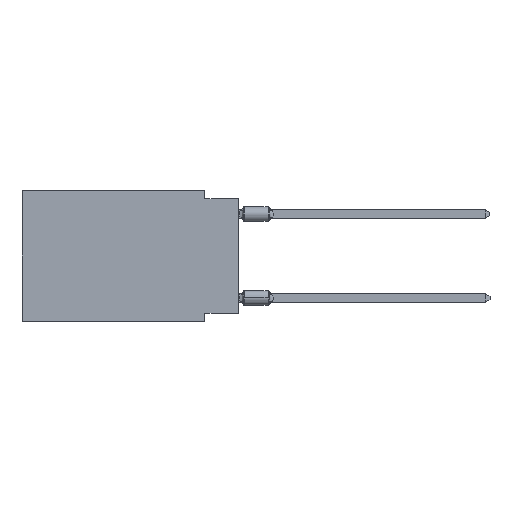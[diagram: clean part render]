
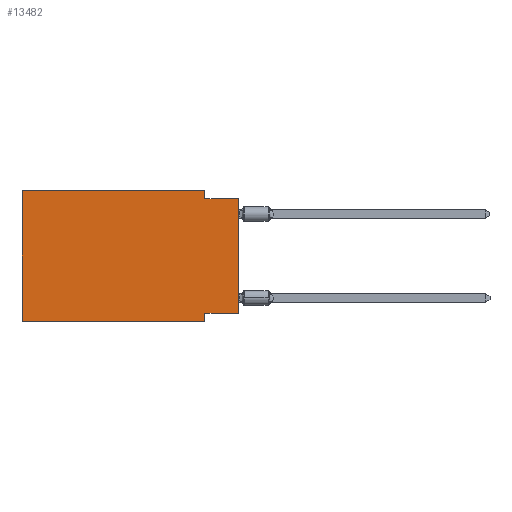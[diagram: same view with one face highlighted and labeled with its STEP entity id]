
A CAD part, left-side view. The second image highlights one B-rep face of the part: STEP entity #13482.
In plain terms, the highlighted planar face has unit normal (-1, 0, 0).
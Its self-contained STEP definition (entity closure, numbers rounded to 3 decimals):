
#192 = VECTOR ( 'NONE', #12420, 1000. ) ;
#428 = FACE_OUTER_BOUND ( 'NONE', #1372, .T. ) ;
#1372 = EDGE_LOOP ( 'NONE', ( #19660, #2529, #6090, #4641, #7979, #2381, #9704, #11062 ) ) ;
#2066 = DIRECTION ( 'NONE',  ( 0., 0., -1. ) ) ;
#2113 = CARTESIAN_POINT ( 'NONE',  ( 0., 16.383, -9.906 ) ) ;
#2270 = CARTESIAN_POINT ( 'NONE',  ( 0., 0., -9.271 ) ) ;
#2381 = ORIENTED_EDGE ( 'NONE', *, *, #20082, .T. ) ;
#2529 = ORIENTED_EDGE ( 'NONE', *, *, #18034, .F. ) ;
#2822 = LINE ( 'NONE', #4248, #22181 ) ;
#3135 = CARTESIAN_POINT ( 'NONE',  ( 0., 0., -9.271 ) ) ;
#3414 = VERTEX_POINT ( 'NONE', #22710 ) ;
#3429 = CARTESIAN_POINT ( 'NONE',  ( 0., 16.383, 0. ) ) ;
#3911 = VERTEX_POINT ( 'NONE', #24845 ) ;
#4010 = VECTOR ( 'NONE', #24298, 1000. ) ;
#4248 = CARTESIAN_POINT ( 'NONE',  ( 0., 16.383, 0. ) ) ;
#4368 = VERTEX_POINT ( 'NONE', #13563 ) ;
#4641 = ORIENTED_EDGE ( 'NONE', *, *, #23853, .F. ) ;
#4750 = CARTESIAN_POINT ( 'NONE',  ( 0., 0., -0.635 ) ) ;
#5993 = LINE ( 'NONE', #15345, #20085 ) ;
#6090 = ORIENTED_EDGE ( 'NONE', *, *, #12623, .F. ) ;
#7596 = EDGE_CURVE ( 'NONE', #4368, #17923, #5993, .T. ) ;
#7607 = VERTEX_POINT ( 'NONE', #21275 ) ;
#7979 = ORIENTED_EDGE ( 'NONE', *, *, #21649, .F. ) ;
#7995 = VECTOR ( 'NONE', #15087, 1000. ) ;
#8327 = PLANE ( 'NONE',  #20786 ) ;
#8394 = CARTESIAN_POINT ( 'NONE',  ( 0., 0., 0. ) ) ;
#8769 = VERTEX_POINT ( 'NONE', #2113 ) ;
#9667 = VERTEX_POINT ( 'NONE', #2270 ) ;
#9704 = ORIENTED_EDGE ( 'NONE', *, *, #7596, .F. ) ;
#11062 = ORIENTED_EDGE ( 'NONE', *, *, #13588, .F. ) ;
#11653 = VERTEX_POINT ( 'NONE', #18395 ) ;
#11945 = DIRECTION ( 'NONE',  ( 1., 0., 0. ) ) ;
#12274 = LINE ( 'NONE', #8394, #4010 ) ;
#12420 = DIRECTION ( 'NONE',  ( 0., -1., 0. ) ) ;
#12623 = EDGE_CURVE ( 'NONE', #3414, #11653, #13606, .T. ) ;
#12642 = DIRECTION ( 'NONE',  ( 0., -1., 0. ) ) ;
#13482 = ADVANCED_FACE ( 'NONE', ( #428 ), #8327, .F. ) ;
#13563 = CARTESIAN_POINT ( 'NONE',  ( 0., 2.54, -9.271 ) ) ;
#13588 = EDGE_CURVE ( 'NONE', #9667, #4368, #18662, .T. ) ;
#13606 = LINE ( 'NONE', #19672, #23616 ) ;
#13886 = CARTESIAN_POINT ( 'NONE',  ( 0., 16.383, 0. ) ) ;
#14705 = VECTOR ( 'NONE', #12642, 1000. ) ;
#15087 = DIRECTION ( 'NONE',  ( 0., 0., 1. ) ) ;
#15345 = CARTESIAN_POINT ( 'NONE',  ( 0., 2.54, -9.906 ) ) ;
#16920 = CARTESIAN_POINT ( 'NONE',  ( 0., 2.54, -9.906 ) ) ;
#17923 = VERTEX_POINT ( 'NONE', #16920 ) ;
#18034 = EDGE_CURVE ( 'NONE', #11653, #3911, #22461, .T. ) ;
#18355 = CARTESIAN_POINT ( 'NONE',  ( 0., 16.383, -9.906 ) ) ;
#18395 = CARTESIAN_POINT ( 'NONE',  ( 0., 2.54, -0.635 ) ) ;
#18403 = DIRECTION ( 'NONE',  ( 0., 1., 0. ) ) ;
#18480 = DIRECTION ( 'NONE',  ( 0., -1., 0. ) ) ;
#18662 = LINE ( 'NONE', #3135, #21587 ) ;
#19660 = ORIENTED_EDGE ( 'NONE', *, *, #23935, .T. ) ;
#19672 = CARTESIAN_POINT ( 'NONE',  ( 0., 2.54, 0. ) ) ;
#19714 = DIRECTION ( 'NONE',  ( 0., 0., -1. ) ) ;
#20082 = EDGE_CURVE ( 'NONE', #8769, #17923, #22238, .T. ) ;
#20085 = VECTOR ( 'NONE', #19714, 1000. ) ;
#20786 = AXIS2_PLACEMENT_3D ( 'NONE', #13886, #11945, #21904 ) ;
#21157 = LINE ( 'NONE', #3429, #7995 ) ;
#21275 = CARTESIAN_POINT ( 'NONE',  ( 0., 16.383, 0. ) ) ;
#21587 = VECTOR ( 'NONE', #18403, 1000. ) ;
#21649 = EDGE_CURVE ( 'NONE', #8769, #7607, #21157, .T. ) ;
#21904 = DIRECTION ( 'NONE',  ( 0., 0., -1. ) ) ;
#22181 = VECTOR ( 'NONE', #18480, 1000. ) ;
#22238 = LINE ( 'NONE', #18355, #192 ) ;
#22461 = LINE ( 'NONE', #4750, #14705 ) ;
#22710 = CARTESIAN_POINT ( 'NONE',  ( 0., 2.54, 0. ) ) ;
#23616 = VECTOR ( 'NONE', #2066, 1000. ) ;
#23853 = EDGE_CURVE ( 'NONE', #7607, #3414, #2822, .T. ) ;
#23935 = EDGE_CURVE ( 'NONE', #9667, #3911, #12274, .T. ) ;
#24298 = DIRECTION ( 'NONE',  ( 0., 0., 1. ) ) ;
#24845 = CARTESIAN_POINT ( 'NONE',  ( 0., 0., -0.635 ) ) ;
